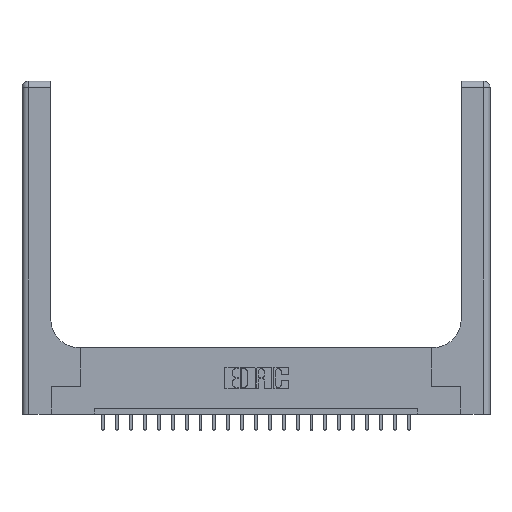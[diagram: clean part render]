
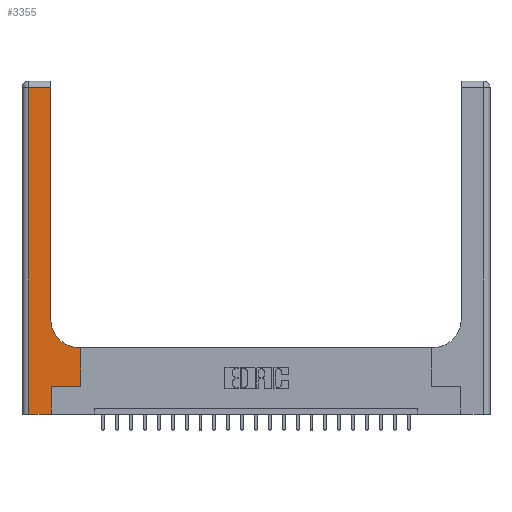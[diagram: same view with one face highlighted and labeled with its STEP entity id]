
A CAD part, top view. The second image highlights one B-rep face of the part: STEP entity #3355.
In plain terms, the highlighted planar face has unit normal (0, 0, 1).
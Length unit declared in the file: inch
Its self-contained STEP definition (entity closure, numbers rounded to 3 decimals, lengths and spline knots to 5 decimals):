
#87 = EDGE_CURVE ( 'NONE', #2745, #5371, #20718, .T. ) ;
#363 = EDGE_CURVE ( 'NONE', #11887, #15717, #6887, .T. ) ;
#413 = CARTESIAN_POINT ( 'NONE',  ( 0.26, 3., 0.37 ) ) ;
#462 = CARTESIAN_POINT ( 'NONE',  ( 0.265, 0., 0.37 ) ) ;
#1087 = ORIENTED_EDGE ( 'NONE', *, *, #363, .T. ) ;
#1200 = VERTEX_POINT ( 'NONE', #18231 ) ;
#1333 = VECTOR ( 'NONE', #7695, 39.37008 ) ;
#1636 = DIRECTION ( 'NONE',  ( 1., 0., 0. ) ) ;
#1956 = ORIENTED_EDGE ( 'NONE', *, *, #2917, .T. ) ;
#2351 = CARTESIAN_POINT ( 'NONE',  ( 0.528, 0.6, 0.37 ) ) ;
#2370 = VECTOR ( 'NONE', #8412, 39.37008 ) ;
#2439 = DIRECTION ( 'NONE',  ( 1., 0., 0. ) ) ;
#2745 = VERTEX_POINT ( 'NONE', #2351 ) ;
#2917 = EDGE_CURVE ( 'NONE', #5371, #21913, #16400, .T. ) ;
#3355 = ADVANCED_FACE ( 'NONE', ( #5986 ), #7874, .F. ) ;
#3705 = VECTOR ( 'NONE', #13319, 39.37008 ) ;
#4440 = VERTEX_POINT ( 'NONE', #4927 ) ;
#4509 = VERTEX_POINT ( 'NONE', #15650 ) ;
#4742 = CARTESIAN_POINT ( 'NONE',  ( 0.265, 0.25, 0.37 ) ) ;
#4766 = VECTOR ( 'NONE', #11347, 39.37008 ) ;
#4927 = CARTESIAN_POINT ( 'NONE',  ( 0.06, 0., 0.37 ) ) ;
#5371 = VERTEX_POINT ( 'NONE', #11278 ) ;
#5373 = LINE ( 'NONE', #21239, #8837 ) ;
#5581 = VECTOR ( 'NONE', #2439, 39.37008 ) ;
#5801 = AXIS2_PLACEMENT_3D ( 'NONE', #12968, #21203, #14391 ) ;
#5986 = FACE_OUTER_BOUND ( 'NONE', #21976, .T. ) ;
#6236 = DIRECTION ( 'NONE',  ( 0., 1., 0. ) ) ;
#6385 = CARTESIAN_POINT ( 'NONE',  ( 0.26, 2.94, 0.37 ) ) ;
#6470 = EDGE_CURVE ( 'NONE', #4509, #2745, #5373, .T. ) ;
#6887 = LINE ( 'NONE', #16678, #2370 ) ;
#7600 = VERTEX_POINT ( 'NONE', #6385 ) ;
#7695 = DIRECTION ( 'NONE',  ( 0., -1., 0. ) ) ;
#7874 = PLANE ( 'NONE',  #5801 ) ;
#7974 = ORIENTED_EDGE ( 'NONE', *, *, #20587, .T. ) ;
#8055 = CARTESIAN_POINT ( 'NONE',  ( 0.26, 0.85, 0.37 ) ) ;
#8228 = LINE ( 'NONE', #21760, #3705 ) ;
#8262 = ORIENTED_EDGE ( 'NONE', *, *, #6470, .T. ) ;
#8412 = DIRECTION ( 'NONE',  ( 0., 1., 0. ) ) ;
#8837 = VECTOR ( 'NONE', #6236, 39.37008 ) ;
#9175 = CARTESIAN_POINT ( 'NONE',  ( 0.265, 0.25, 0.37 ) ) ;
#9305 = ORIENTED_EDGE ( 'NONE', *, *, #20347, .T. ) ;
#9360 = LINE ( 'NONE', #14505, #1333 ) ;
#10133 = LINE ( 'NONE', #12813, #5581 ) ;
#11266 = EDGE_CURVE ( 'NONE', #15717, #4509, #19207, .T. ) ;
#11278 = CARTESIAN_POINT ( 'NONE',  ( 0.51, 0.6, 0.37 ) ) ;
#11347 = DIRECTION ( 'NONE',  ( -1., 0., 0. ) ) ;
#11887 = VERTEX_POINT ( 'NONE', #462 ) ;
#12283 = DIRECTION ( 'NONE',  ( 0., 1., 0. ) ) ;
#12813 = CARTESIAN_POINT ( 'NONE',  ( 0., 0., 0.37 ) ) ;
#12968 = CARTESIAN_POINT ( 'NONE',  ( 0., 3., 0.37 ) ) ;
#13143 = VECTOR ( 'NONE', #20050, 39.37008 ) ;
#13319 = DIRECTION ( 'NONE',  ( -1., 0., 0. ) ) ;
#14391 = DIRECTION ( 'NONE',  ( -1., 0., 0. ) ) ;
#14505 = CARTESIAN_POINT ( 'NONE',  ( 0.06, 3., 0.37 ) ) ;
#14993 = VECTOR ( 'NONE', #12283, 39.37008 ) ;
#15650 = CARTESIAN_POINT ( 'NONE',  ( 0.528, 0.25, 0.37 ) ) ;
#15717 = VERTEX_POINT ( 'NONE', #9175 ) ;
#15841 = CARTESIAN_POINT ( 'NONE',  ( 0.51, 0.85, 0.37 ) ) ;
#16390 = EDGE_CURVE ( 'NONE', #4440, #11887, #10133, .T. ) ;
#16400 = CIRCLE ( 'NONE', #17938, 0.25 ) ;
#16439 = ORIENTED_EDGE ( 'NONE', *, *, #87, .T. ) ;
#16517 = EDGE_CURVE ( 'NONE', #7600, #1200, #8228, .T. ) ;
#16678 = CARTESIAN_POINT ( 'NONE',  ( 0.265, 0., 0.37 ) ) ;
#16700 = DIRECTION ( 'NONE',  ( 0., 0., -1. ) ) ;
#17113 = ORIENTED_EDGE ( 'NONE', *, *, #16390, .T. ) ;
#17938 = AXIS2_PLACEMENT_3D ( 'NONE', #15841, #16700, #1636 ) ;
#18231 = CARTESIAN_POINT ( 'NONE',  ( 0.06, 2.94, 0.37 ) ) ;
#19207 = LINE ( 'NONE', #4742, #13143 ) ;
#20050 = DIRECTION ( 'NONE',  ( 1., 0., 0. ) ) ;
#20276 = LINE ( 'NONE', #413, #14993 ) ;
#20346 = ORIENTED_EDGE ( 'NONE', *, *, #11266, .T. ) ;
#20347 = EDGE_CURVE ( 'NONE', #21913, #7600, #20276, .T. ) ;
#20587 = EDGE_CURVE ( 'NONE', #1200, #4440, #9360, .T. ) ;
#20718 = LINE ( 'NONE', #21285, #4766 ) ;
#21203 = DIRECTION ( 'NONE',  ( 0., 0., -1. ) ) ;
#21207 = ORIENTED_EDGE ( 'NONE', *, *, #16517, .T. ) ;
#21239 = CARTESIAN_POINT ( 'NONE',  ( 0.528, 0.25, 0.37 ) ) ;
#21285 = CARTESIAN_POINT ( 'NONE',  ( 0.26, 0.6, 0.37 ) ) ;
#21760 = CARTESIAN_POINT ( 'NONE',  ( 0., 2.94, 0.37 ) ) ;
#21913 = VERTEX_POINT ( 'NONE', #8055 ) ;
#21976 = EDGE_LOOP ( 'NONE', ( #9305, #21207, #7974, #17113, #1087, #20346, #8262, #16439, #1956 ) ) ;
